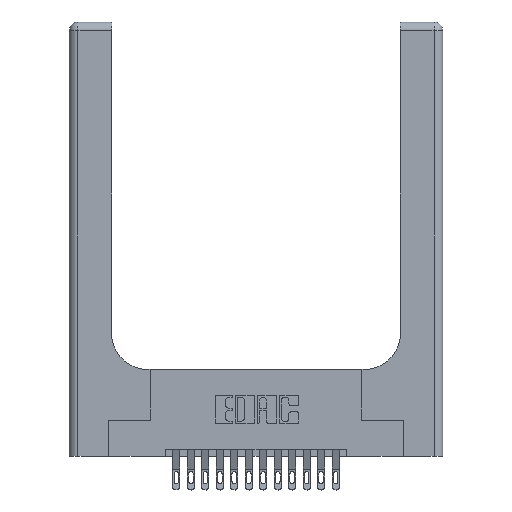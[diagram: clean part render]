
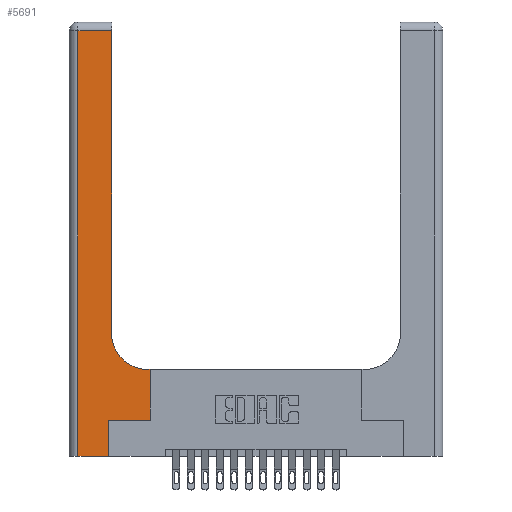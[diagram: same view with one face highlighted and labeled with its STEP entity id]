
A CAD part, top view. The second image highlights one B-rep face of the part: STEP entity #5691.
In plain terms, the highlighted planar face has unit normal (0, 0, 1).
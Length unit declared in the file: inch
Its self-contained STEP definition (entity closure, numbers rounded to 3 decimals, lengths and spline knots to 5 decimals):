
#285 = VECTOR ( 'NONE', #2643, 39.37008 ) ;
#397 = CARTESIAN_POINT ( 'NONE',  ( 0.269, 0., 0.37 ) ) ;
#482 = DIRECTION ( 'NONE',  ( 1., 0., 0. ) ) ;
#514 = CARTESIAN_POINT ( 'NONE',  ( 0.5585, 0.25, 0.37 ) ) ;
#656 = EDGE_CURVE ( 'NONE', #14730, #6566, #2961, .T. ) ;
#987 = CARTESIAN_POINT ( 'NONE',  ( 0., 0., 0.37 ) ) ;
#1224 = CARTESIAN_POINT ( 'NONE',  ( 0.2915, 0.6, 0.37 ) ) ;
#1257 = CARTESIAN_POINT ( 'NONE',  ( 0.5585, 0.6, 0.37 ) ) ;
#1527 = CARTESIAN_POINT ( 'NONE',  ( 0.2915, 2.94, 0.37 ) ) ;
#1637 = EDGE_CURVE ( 'NONE', #6566, #13119, #7964, .T. ) ;
#1682 = ORIENTED_EDGE ( 'NONE', *, *, #1637, .T. ) ;
#1735 = VERTEX_POINT ( 'NONE', #1257 ) ;
#1823 = FACE_OUTER_BOUND ( 'NONE', #12300, .T. ) ;
#2383 = PLANE ( 'NONE',  #4129 ) ;
#2643 = DIRECTION ( 'NONE',  ( -1., 0., 0. ) ) ;
#2961 = LINE ( 'NONE', #10633, #7773 ) ;
#3619 = VERTEX_POINT ( 'NONE', #1527 ) ;
#3673 = LINE ( 'NONE', #3753, #7600 ) ;
#3753 = CARTESIAN_POINT ( 'NONE',  ( 0.5585, 0.25, 0.37 ) ) ;
#3810 = DIRECTION ( 'NONE',  ( 0., 1., 0. ) ) ;
#3866 = DIRECTION ( 'NONE',  ( 0., 0., -1. ) ) ;
#3900 = CARTESIAN_POINT ( 'NONE',  ( 0.06, 0., 0.37 ) ) ;
#4129 = AXIS2_PLACEMENT_3D ( 'NONE', #6640, #3866, #8107 ) ;
#4175 = LINE ( 'NONE', #1224, #285 ) ;
#5117 = EDGE_CURVE ( 'NONE', #18546, #15562, #17508, .T. ) ;
#5218 = AXIS2_PLACEMENT_3D ( 'NONE', #10652, #13640, #482 ) ;
#5517 = EDGE_CURVE ( 'NONE', #9253, #1735, #3673, .T. ) ;
#5555 = VECTOR ( 'NONE', #13542, 39.37008 ) ;
#5691 = ADVANCED_FACE ( 'NONE', ( #1823 ), #2383, .F. ) ;
#6276 = EDGE_CURVE ( 'NONE', #12454, #9253, #12309, .T. ) ;
#6454 = DIRECTION ( 'NONE',  ( -1., 0., 0. ) ) ;
#6566 = VERTEX_POINT ( 'NONE', #3900 ) ;
#6640 = CARTESIAN_POINT ( 'NONE',  ( 0., 3., 0.37 ) ) ;
#6777 = VECTOR ( 'NONE', #6454, 39.37008 ) ;
#7249 = DIRECTION ( 'NONE',  ( 1., 0., 0. ) ) ;
#7600 = VECTOR ( 'NONE', #3810, 39.37008 ) ;
#7773 = VECTOR ( 'NONE', #17952, 39.37008 ) ;
#7825 = LINE ( 'NONE', #10374, #13312 ) ;
#7964 = LINE ( 'NONE', #987, #14363 ) ;
#8107 = DIRECTION ( 'NONE',  ( -1., 0., 0. ) ) ;
#8216 = EDGE_CURVE ( 'NONE', #3619, #14730, #12954, .T. ) ;
#8509 = ORIENTED_EDGE ( 'NONE', *, *, #5117, .T. ) ;
#9011 = CARTESIAN_POINT ( 'NONE',  ( 0.269, 0.25, 0.37 ) ) ;
#9253 = VERTEX_POINT ( 'NONE', #514 ) ;
#9818 = CARTESIAN_POINT ( 'NONE',  ( 0.5415, 0.6, 0.37 ) ) ;
#10374 = CARTESIAN_POINT ( 'NONE',  ( 0.2915, 3., 0.37 ) ) ;
#10633 = CARTESIAN_POINT ( 'NONE',  ( 0.06, 3., 0.37 ) ) ;
#10652 = CARTESIAN_POINT ( 'NONE',  ( 0.5415, 0.85, 0.37 ) ) ;
#10904 = ORIENTED_EDGE ( 'NONE', *, *, #5517, .T. ) ;
#12000 = EDGE_CURVE ( 'NONE', #13119, #12454, #13320, .T. ) ;
#12219 = ORIENTED_EDGE ( 'NONE', *, *, #8216, .T. ) ;
#12300 = EDGE_LOOP ( 'NONE', ( #13672, #12219, #13745, #1682, #17223, #12439, #10904, #16291, #8509 ) ) ;
#12309 = LINE ( 'NONE', #9011, #17144 ) ;
#12439 = ORIENTED_EDGE ( 'NONE', *, *, #6276, .T. ) ;
#12454 = VERTEX_POINT ( 'NONE', #17732 ) ;
#12952 = EDGE_CURVE ( 'NONE', #1735, #18546, #4175, .T. ) ;
#12954 = LINE ( 'NONE', #13718, #6777 ) ;
#13119 = VERTEX_POINT ( 'NONE', #397 ) ;
#13233 = DIRECTION ( 'NONE',  ( 0., 1., 0. ) ) ;
#13312 = VECTOR ( 'NONE', #13233, 39.37008 ) ;
#13320 = LINE ( 'NONE', #16430, #5555 ) ;
#13542 = DIRECTION ( 'NONE',  ( 0., 1., 0. ) ) ;
#13640 = DIRECTION ( 'NONE',  ( 0., 0., -1. ) ) ;
#13672 = ORIENTED_EDGE ( 'NONE', *, *, #14147, .T. ) ;
#13718 = CARTESIAN_POINT ( 'NONE',  ( 0., 2.94, 0.37 ) ) ;
#13745 = ORIENTED_EDGE ( 'NONE', *, *, #656, .T. ) ;
#14147 = EDGE_CURVE ( 'NONE', #15562, #3619, #7825, .T. ) ;
#14363 = VECTOR ( 'NONE', #7249, 39.37008 ) ;
#14730 = VERTEX_POINT ( 'NONE', #17584 ) ;
#15205 = CARTESIAN_POINT ( 'NONE',  ( 0.2915, 0.85, 0.37 ) ) ;
#15562 = VERTEX_POINT ( 'NONE', #15205 ) ;
#16150 = DIRECTION ( 'NONE',  ( 1., 0., 0. ) ) ;
#16291 = ORIENTED_EDGE ( 'NONE', *, *, #12952, .T. ) ;
#16430 = CARTESIAN_POINT ( 'NONE',  ( 0.269, 0., 0.37 ) ) ;
#17144 = VECTOR ( 'NONE', #16150, 39.37008 ) ;
#17223 = ORIENTED_EDGE ( 'NONE', *, *, #12000, .T. ) ;
#17508 = CIRCLE ( 'NONE', #5218, 0.25 ) ;
#17584 = CARTESIAN_POINT ( 'NONE',  ( 0.06, 2.94, 0.37 ) ) ;
#17732 = CARTESIAN_POINT ( 'NONE',  ( 0.269, 0.25, 0.37 ) ) ;
#17952 = DIRECTION ( 'NONE',  ( 0., -1., 0. ) ) ;
#18546 = VERTEX_POINT ( 'NONE', #9818 ) ;
